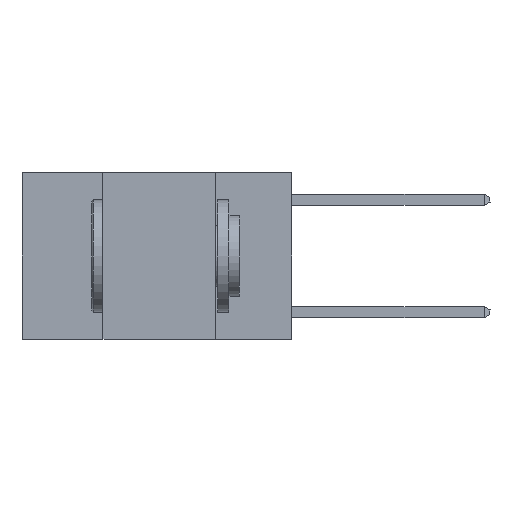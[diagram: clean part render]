
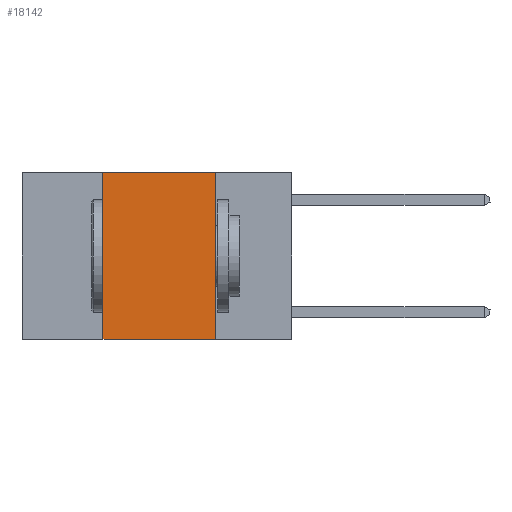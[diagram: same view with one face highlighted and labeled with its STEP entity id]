
A CAD part, left-side view. The second image highlights one B-rep face of the part: STEP entity #18142.
In plain terms, the highlighted planar face has unit normal (-1, 0, 0).
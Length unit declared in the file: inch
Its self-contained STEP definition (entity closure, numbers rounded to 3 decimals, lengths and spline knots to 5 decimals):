
#532 = CARTESIAN_POINT ( 'NONE',  ( 0., 0.17, -0.37 ) ) ;
#599 = DIRECTION ( 'NONE',  ( 0., -1., 0. ) ) ;
#1299 = FACE_OUTER_BOUND ( 'NONE', #3609, .T. ) ;
#1476 = DIRECTION ( 'NONE',  ( 0., 0., -1. ) ) ;
#1702 = CARTESIAN_POINT ( 'NONE',  ( 0., 0.42, 0. ) ) ;
#3308 = VECTOR ( 'NONE', #9948, 39.37008 ) ;
#3609 = EDGE_LOOP ( 'NONE', ( #4193, #4599, #4623, #4662 ) ) ;
#4193 = ORIENTED_EDGE ( 'NONE', *, *, #8683, .F. ) ;
#4418 = VERTEX_POINT ( 'NONE', #12825 ) ;
#4599 = ORIENTED_EDGE ( 'NONE', *, *, #8450, .F. ) ;
#4623 = ORIENTED_EDGE ( 'NONE', *, *, #16001, .F. ) ;
#4662 = ORIENTED_EDGE ( 'NONE', *, *, #11011, .T. ) ;
#4945 = CARTESIAN_POINT ( 'NONE',  ( 0., 0.6, 0. ) ) ;
#5438 = LINE ( 'NONE', #17789, #18937 ) ;
#6031 = DIRECTION ( 'NONE',  ( 0., 0., 1. ) ) ;
#7849 = CARTESIAN_POINT ( 'NONE',  ( 0., 0.42, -0.37 ) ) ;
#8332 = LINE ( 'NONE', #13019, #13636 ) ;
#8450 = EDGE_CURVE ( 'NONE', #9569, #4418, #8332, .T. ) ;
#8683 = EDGE_CURVE ( 'NONE', #4418, #20587, #21878, .T. ) ;
#9569 = VERTEX_POINT ( 'NONE', #1702 ) ;
#9948 = DIRECTION ( 'NONE',  ( 0., 0., -1. ) ) ;
#10749 = DIRECTION ( 'NONE',  ( 0., -1., 0. ) ) ;
#11011 = EDGE_CURVE ( 'NONE', #11812, #20587, #5438, .T. ) ;
#11812 = VERTEX_POINT ( 'NONE', #7849 ) ;
#12127 = DIRECTION ( 'NONE',  ( 1., 0., 0. ) ) ;
#12825 = CARTESIAN_POINT ( 'NONE',  ( 0., 0.17, 0. ) ) ;
#13019 = CARTESIAN_POINT ( 'NONE',  ( 0., 0.6, 0. ) ) ;
#13636 = VECTOR ( 'NONE', #599, 39.37008 ) ;
#13677 = VECTOR ( 'NONE', #6031, 39.37008 ) ;
#16001 = EDGE_CURVE ( 'NONE', #11812, #9569, #18273, .T. ) ;
#17789 = CARTESIAN_POINT ( 'NONE',  ( 0., 0.6, -0.37 ) ) ;
#18142 = ADVANCED_FACE ( 'NONE', ( #1299 ), #22360, .F. ) ;
#18273 = LINE ( 'NONE', #21625, #13677 ) ;
#18937 = VECTOR ( 'NONE', #10749, 39.37008 ) ;
#19890 = AXIS2_PLACEMENT_3D ( 'NONE', #4945, #12127, #1476 ) ;
#20587 = VERTEX_POINT ( 'NONE', #532 ) ;
#21625 = CARTESIAN_POINT ( 'NONE',  ( 0., 0.42, 0. ) ) ;
#21878 = LINE ( 'NONE', #22104, #3308 ) ;
#22104 = CARTESIAN_POINT ( 'NONE',  ( 0., 0.17, 0. ) ) ;
#22360 = PLANE ( 'NONE',  #19890 ) ;
